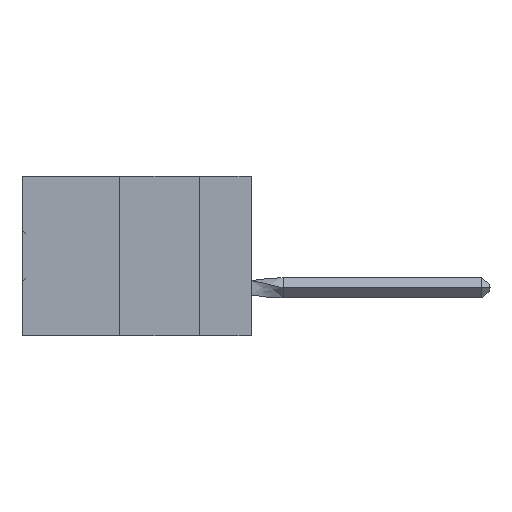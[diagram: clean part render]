
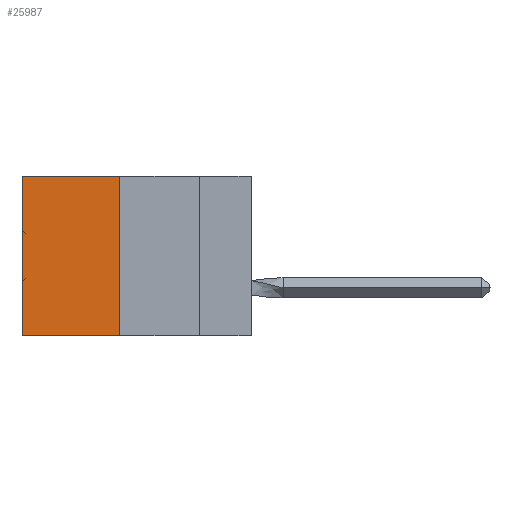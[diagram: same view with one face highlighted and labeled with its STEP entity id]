
A CAD part, left-side view. The second image highlights one B-rep face of the part: STEP entity #25987.
In plain terms, the highlighted planar face has unit normal (-1, 0, 0).
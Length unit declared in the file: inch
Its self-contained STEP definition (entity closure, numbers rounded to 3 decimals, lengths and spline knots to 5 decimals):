
#5774 = ORIENTED_EDGE ( 'NONE', *, *, #38414, .F. ) ;
#10942 = CARTESIAN_POINT ( 'NONE',  ( 0.305, 0.413, 0. ) ) ;
#12552 = DIRECTION ( 'NONE',  ( 0., 1., 0. ) ) ;
#16533 = CARTESIAN_POINT ( 'NONE',  ( 0.305, 0.72, -0.5 ) ) ;
#17175 = DIRECTION ( 'NONE',  ( 0., 0., -1. ) ) ;
#17665 = ORIENTED_EDGE ( 'NONE', *, *, #26762, .F. ) ;
#20376 = LINE ( 'NONE', #23415, #50148 ) ;
#21229 = VERTEX_POINT ( 'NONE', #62749 ) ;
#21909 = LINE ( 'NONE', #55688, #50960 ) ;
#23415 = CARTESIAN_POINT ( 'NONE',  ( 0.305, 0.413, 0. ) ) ;
#25135 = VECTOR ( 'NONE', #12552, 39.37008 ) ;
#25987 = ADVANCED_FACE ( 'NONE', ( #29164 ), #56045, .F. ) ;
#26462 = DIRECTION ( 'NONE',  ( 0., 0., -1. ) ) ;
#26544 = VERTEX_POINT ( 'NONE', #62380 ) ;
#26762 = EDGE_CURVE ( 'NONE', #26544, #49343, #39659, .T. ) ;
#28293 = EDGE_CURVE ( 'NONE', #36017, #21229, #20376, .T. ) ;
#29164 = FACE_OUTER_BOUND ( 'NONE', #36007, .T. ) ;
#31259 = ORIENTED_EDGE ( 'NONE', *, *, #28293, .T. ) ;
#32053 = CARTESIAN_POINT ( 'NONE',  ( 0.305, 0.413, -0.5 ) ) ;
#33351 = DIRECTION ( 'NONE',  ( 0., 1., 0. ) ) ;
#36007 = EDGE_LOOP ( 'NONE', ( #51036, #17665, #5774, #31259 ) ) ;
#36017 = VERTEX_POINT ( 'NONE', #10942 ) ;
#38414 = EDGE_CURVE ( 'NONE', #36017, #26544, #21909, .T. ) ;
#39659 = LINE ( 'NONE', #32053, #25135 ) ;
#41021 = AXIS2_PLACEMENT_3D ( 'NONE', #50520, #60351, #50929 ) ;
#48155 = VECTOR ( 'NONE', #17175, 39.37008 ) ;
#49343 = VERTEX_POINT ( 'NONE', #57631 ) ;
#49871 = EDGE_CURVE ( 'NONE', #21229, #49343, #51939, .T. ) ;
#50148 = VECTOR ( 'NONE', #33351, 39.37008 ) ;
#50520 = CARTESIAN_POINT ( 'NONE',  ( 0.305, 0.413, -0.5 ) ) ;
#50929 = DIRECTION ( 'NONE',  ( 0., 0., -1. ) ) ;
#50960 = VECTOR ( 'NONE', #26462, 39.37008 ) ;
#51036 = ORIENTED_EDGE ( 'NONE', *, *, #49871, .T. ) ;
#51939 = LINE ( 'NONE', #16533, #48155 ) ;
#55688 = CARTESIAN_POINT ( 'NONE',  ( 0.305, 0.413, -0.5 ) ) ;
#56045 = PLANE ( 'NONE',  #41021 ) ;
#57631 = CARTESIAN_POINT ( 'NONE',  ( 0.305, 0.72, -0.5 ) ) ;
#60351 = DIRECTION ( 'NONE',  ( 1., 0., 0. ) ) ;
#62380 = CARTESIAN_POINT ( 'NONE',  ( 0.305, 0.413, -0.5 ) ) ;
#62749 = CARTESIAN_POINT ( 'NONE',  ( 0.305, 0.72, 0. ) ) ;
